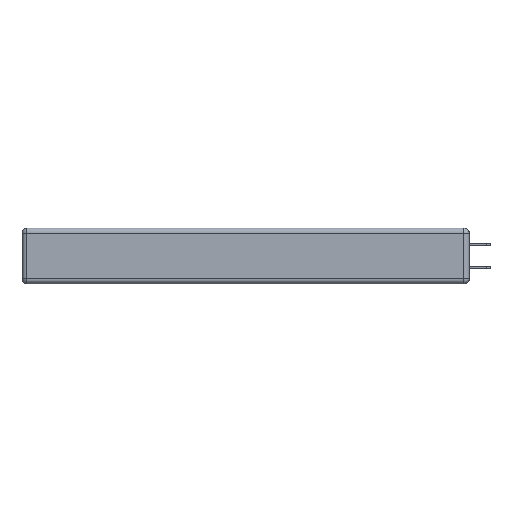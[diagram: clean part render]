
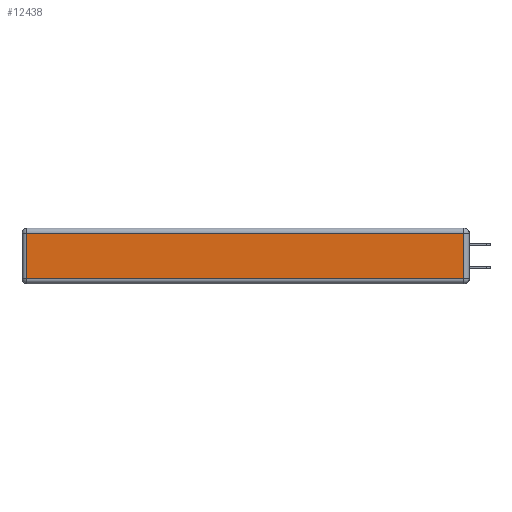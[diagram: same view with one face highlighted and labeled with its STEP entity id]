
A CAD part, left-side view. The second image highlights one B-rep face of the part: STEP entity #12438.
In plain terms, the highlighted planar face has unit normal (-1, 0, 0).
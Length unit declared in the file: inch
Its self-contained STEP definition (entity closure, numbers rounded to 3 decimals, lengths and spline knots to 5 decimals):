
#788 = EDGE_CURVE ( 'NONE', #1896, #7523, #12980, .T. ) ;
#899 = ORIENTED_EDGE ( 'NONE', *, *, #13181, .T. ) ;
#1615 = VECTOR ( 'NONE', #8169, 39.37008 ) ;
#1832 = CARTESIAN_POINT ( 'NONE',  ( 0., 0., -0.343 ) ) ;
#1896 = VERTEX_POINT ( 'NONE', #12140 ) ;
#2012 = VERTEX_POINT ( 'NONE', #7931 ) ;
#2213 = LINE ( 'NONE', #9677, #4847 ) ;
#2337 = EDGE_LOOP ( 'NONE', ( #899, #10527, #8541, #7437 ) ) ;
#3194 = CARTESIAN_POINT ( 'NONE',  ( 0., 0., -0.313 ) ) ;
#3234 = CARTESIAN_POINT ( 'NONE',  ( 0., 2.72, -0.343 ) ) ;
#4847 = VECTOR ( 'NONE', #5321, 39.37008 ) ;
#5321 = DIRECTION ( 'NONE',  ( 0., 1., 0. ) ) ;
#5601 = DIRECTION ( 'NONE',  ( 0., 0., -1. ) ) ;
#6283 = DIRECTION ( 'NONE',  ( 0., 0., 1. ) ) ;
#6829 = FACE_OUTER_BOUND ( 'NONE', #2337, .T. ) ;
#7124 = AXIS2_PLACEMENT_3D ( 'NONE', #1832, #8549, #6283 ) ;
#7437 = ORIENTED_EDGE ( 'NONE', *, *, #11895, .T. ) ;
#7523 = VERTEX_POINT ( 'NONE', #13593 ) ;
#7931 = CARTESIAN_POINT ( 'NONE',  ( 0., 2.72, -0.313 ) ) ;
#8169 = DIRECTION ( 'NONE',  ( 0., 0., 1. ) ) ;
#8541 = ORIENTED_EDGE ( 'NONE', *, *, #9863, .T. ) ;
#8549 = DIRECTION ( 'NONE',  ( -1., 0., 0. ) ) ;
#8759 = LINE ( 'NONE', #3234, #11532 ) ;
#9086 = LINE ( 'NONE', #3194, #12185 ) ;
#9289 = CARTESIAN_POINT ( 'NONE',  ( 0., 2.72, -0.03 ) ) ;
#9677 = CARTESIAN_POINT ( 'NONE',  ( 0., 2.75, -0.03 ) ) ;
#9863 = EDGE_CURVE ( 'NONE', #7523, #13314, #2213, .T. ) ;
#10527 = ORIENTED_EDGE ( 'NONE', *, *, #788, .T. ) ;
#11532 = VECTOR ( 'NONE', #5601, 39.37008 ) ;
#11895 = EDGE_CURVE ( 'NONE', #13314, #2012, #8759, .T. ) ;
#12140 = CARTESIAN_POINT ( 'NONE',  ( 0., 0.03, -0.313 ) ) ;
#12185 = VECTOR ( 'NONE', #14433, 39.37008 ) ;
#12438 = ADVANCED_FACE ( 'NONE', ( #6829 ), #12961, .T. ) ;
#12961 = PLANE ( 'NONE',  #7124 ) ;
#12980 = LINE ( 'NONE', #13238, #1615 ) ;
#13181 = EDGE_CURVE ( 'NONE', #2012, #1896, #9086, .T. ) ;
#13238 = CARTESIAN_POINT ( 'NONE',  ( 0., 0.03, -0.343 ) ) ;
#13314 = VERTEX_POINT ( 'NONE', #9289 ) ;
#13593 = CARTESIAN_POINT ( 'NONE',  ( 0., 0.03, -0.03 ) ) ;
#14433 = DIRECTION ( 'NONE',  ( 0., -1., 0. ) ) ;
